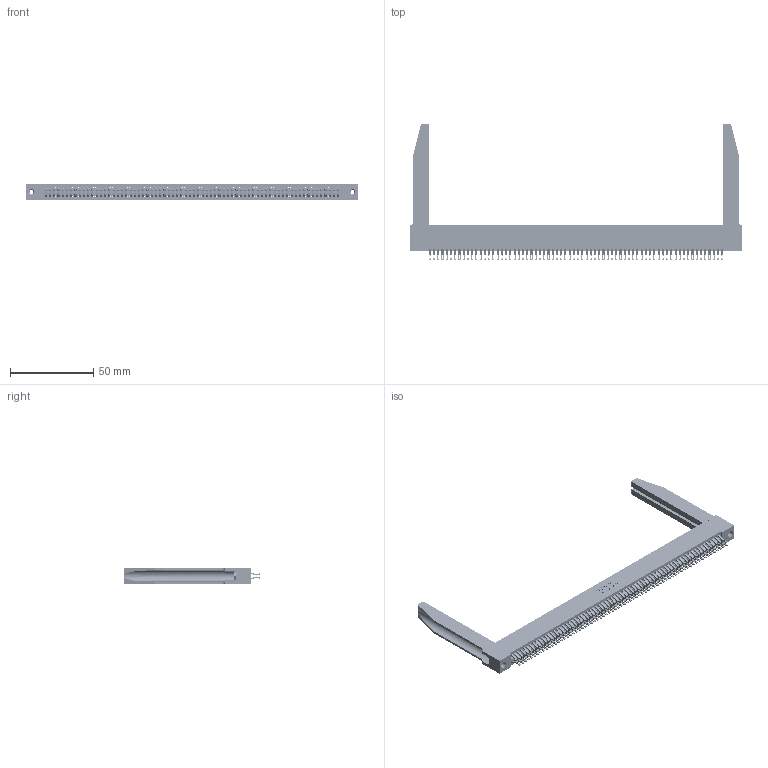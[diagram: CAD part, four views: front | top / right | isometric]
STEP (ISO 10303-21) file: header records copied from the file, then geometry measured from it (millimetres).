
FILE_DESCRIPTION (( 'STEP AP203' ), '1' );
FILE_NAME ('345-140-555-278.STEP', '2019-11-08T22:16:26', ( '' ), ( '' ), 'SwSTEP 2.0', 'SolidWorks 2016', '' );
FILE_SCHEMA (( 'CONFIG_CONTROL_DESIGN' ));
Length unit declared in the file: inch
Products named in the file (5): 345-250-001_345-250-001-102; 345-292-001_555 Tail; 345-140-555-278; 345-220-078_345-220-078; 345 Part_Flush Mounting Lugs - 0.156 Dia-TH
Assembly tree (145 placements, depth 2):
  345-140-555-278
    345 Part_Flush Mounting Lugs - 0.156 Dia-TH
    345-292-001_555 Tail  x140
    345-250-001_345-250-001-102  x2
    345-220-078_345-220-078  x2
Bounding box: 199.03 x 82.09 x 9.4 mm (x, y, z)
Volume: 27770.8 mm3; surface area: 38357.1 mm2
Topology: 145 solids, 145 shells, 8200 faces, 25729 edges, 17142 vertices
Faces by surface type: plane 4562, cylinder 3586, bspline 36, cone 12, torus 4
Entity records: 56220 total; most frequent: CARTESIAN_POINT 10349, ORIENTED_EDGE 9150, DIRECTION 8053, EDGE_CURVE 4575, VECTOR 4049, LINE 4049, VERTEX_POINT 3044, AXIS2_PLACEMENT_3D 2002
